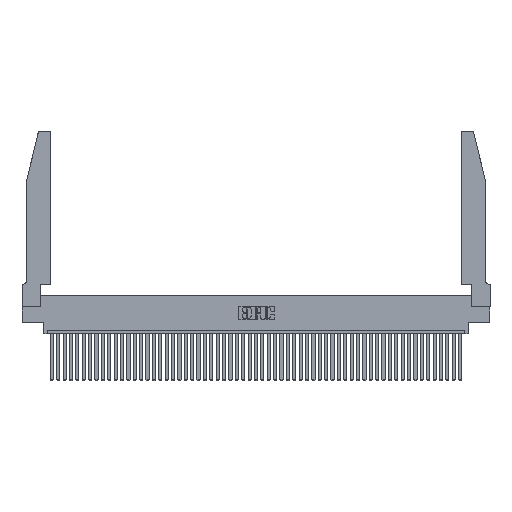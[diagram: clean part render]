
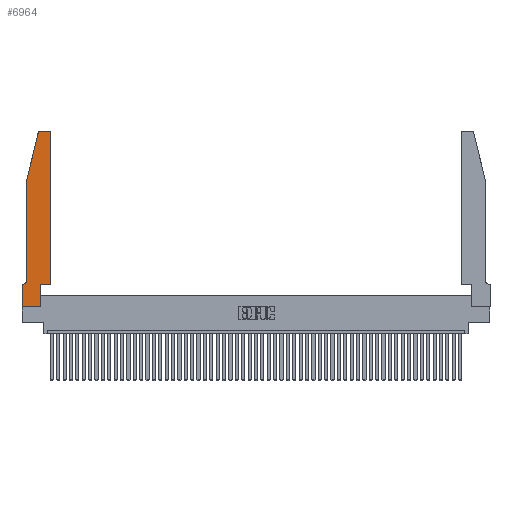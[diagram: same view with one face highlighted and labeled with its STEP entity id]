
A CAD part, top view. The second image highlights one B-rep face of the part: STEP entity #6964.
In plain terms, the highlighted planar face has unit normal (0, 0, 1).
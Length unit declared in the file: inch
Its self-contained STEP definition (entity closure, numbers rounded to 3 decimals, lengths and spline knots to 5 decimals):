
#1527 = DIRECTION ( 'NONE',  ( 0., 1., 0. ) ) ;
#1650 = CARTESIAN_POINT ( 'NONE',  ( 0.2605, 2.75, 0.37 ) ) ;
#1652 = CARTESIAN_POINT ( 'NONE',  ( 0.2865, 0.35, 0.37 ) ) ;
#4080 = VERTEX_POINT ( 'NONE', #32433 ) ;
#4456 = LINE ( 'NONE', #1652, #39812 ) ;
#5148 = CARTESIAN_POINT ( 'NONE',  ( 0., 0., 0.37 ) ) ;
#5754 = EDGE_CURVE ( 'NONE', #23279, #21709, #27894, .T. ) ;
#6207 = CARTESIAN_POINT ( 'NONE',  ( 0.0055, 0.35, 0.37 ) ) ;
#6964 = ADVANCED_FACE ( 'NONE', ( #22169 ), #35498, .T. ) ;
#7252 = VERTEX_POINT ( 'NONE', #6207 ) ;
#7610 = CARTESIAN_POINT ( 'NONE',  ( 0.0755, 2., 0.37 ) ) ;
#8120 = LINE ( 'NONE', #5148, #44692 ) ;
#9779 = VERTEX_POINT ( 'NONE', #18136 ) ;
#9896 = LINE ( 'NONE', #1650, #31781 ) ;
#10762 = VERTEX_POINT ( 'NONE', #33811 ) ;
#10920 = VERTEX_POINT ( 'NONE', #19626 ) ;
#11100 = VERTEX_POINT ( 'NONE', #49220 ) ;
#11203 = DIRECTION ( 'NONE',  ( -0.239, -0.971, 0. ) ) ;
#11654 = VECTOR ( 'NONE', #16954, 39.37008 ) ;
#11927 = CARTESIAN_POINT ( 'NONE',  ( 0.4505, 0.35, 0.37 ) ) ;
#12355 = VECTOR ( 'NONE', #30976, 39.37008 ) ;
#12578 = CARTESIAN_POINT ( 'NONE',  ( 0.0755, 0.35, 0.37 ) ) ;
#13066 = EDGE_CURVE ( 'NONE', #10920, #11100, #47087, .T. ) ;
#13145 = EDGE_CURVE ( 'NONE', #11100, #16964, #33066, .T. ) ;
#13948 = CIRCLE ( 'NONE', #41831, 0.07 ) ;
#14641 = ORIENTED_EDGE ( 'NONE', *, *, #19380, .T. ) ;
#15115 = DIRECTION ( 'NONE',  ( 0., 0., 1. ) ) ;
#15312 = LINE ( 'NONE', #50523, #23232 ) ;
#15313 = EDGE_LOOP ( 'NONE', ( #14641, #48145, #34762, #48092, #24814, #31994, #47638, #49936, #45730, #36715, #20495, #25054 ) ) ;
#15328 = EDGE_CURVE ( 'NONE', #36729, #23279, #18245, .T. ) ;
#15390 = DIRECTION ( 'NONE',  ( 1., 0., 0. ) ) ;
#16580 = VERTEX_POINT ( 'NONE', #29327 ) ;
#16954 = DIRECTION ( 'NONE',  ( -1., 0., 0. ) ) ;
#16964 = VERTEX_POINT ( 'NONE', #40694 ) ;
#16965 = CARTESIAN_POINT ( 'NONE',  ( 0.0755, 2., 0.37 ) ) ;
#17704 = CARTESIAN_POINT ( 'NONE',  ( 0.25487, 2.72718, 0.37 ) ) ;
#18136 = CARTESIAN_POINT ( 'NONE',  ( 0.0755, 0.42, 0.37 ) ) ;
#18245 = CIRCLE ( 'NONE', #34165, 0.03 ) ;
#18463 = DIRECTION ( 'NONE',  ( 0., 0., 1. ) ) ;
#19380 = EDGE_CURVE ( 'NONE', #16964, #36729, #9896, .T. ) ;
#19626 = CARTESIAN_POINT ( 'NONE',  ( 0.4505, 0.35, 0.37 ) ) ;
#20127 = DIRECTION ( 'NONE',  ( 1., 0., 0. ) ) ;
#20192 = CARTESIAN_POINT ( 'NONE',  ( 0., 0., 0.37 ) ) ;
#20495 = ORIENTED_EDGE ( 'NONE', *, *, #13066, .T. ) ;
#20554 = CARTESIAN_POINT ( 'NONE',  ( 0.4505, 0.35, 0.37 ) ) ;
#21009 = DIRECTION ( 'NONE',  ( 0., -1., 0. ) ) ;
#21709 = VERTEX_POINT ( 'NONE', #16965 ) ;
#21934 = VERTEX_POINT ( 'NONE', #20192 ) ;
#22025 = LINE ( 'NONE', #12578, #11654 ) ;
#22169 = FACE_OUTER_BOUND ( 'NONE', #15313, .T. ) ;
#23232 = VECTOR ( 'NONE', #15390, 39.37008 ) ;
#23279 = VERTEX_POINT ( 'NONE', #17704 ) ;
#23739 = CARTESIAN_POINT ( 'NONE',  ( 0.0755, 2., 0.37 ) ) ;
#24238 = DIRECTION ( 'NONE',  ( 0., 0., 1. ) ) ;
#24558 = EDGE_CURVE ( 'NONE', #21709, #9779, #44012, .T. ) ;
#24789 = DIRECTION ( 'NONE',  ( 0., 1., 0. ) ) ;
#24814 = ORIENTED_EDGE ( 'NONE', *, *, #33190, .T. ) ;
#25054 = ORIENTED_EDGE ( 'NONE', *, *, #13145, .T. ) ;
#25460 = VECTOR ( 'NONE', #11203, 39.37008 ) ;
#26662 = DIRECTION ( 'NONE',  ( 1., 0., 0. ) ) ;
#27894 = LINE ( 'NONE', #7610, #25460 ) ;
#27933 = EDGE_CURVE ( 'NONE', #16580, #21934, #8120, .T. ) ;
#28600 = CARTESIAN_POINT ( 'NONE',  ( 0.284, 2.75, 0.37 ) ) ;
#29327 = CARTESIAN_POINT ( 'NONE',  ( 0., 0.35, 0.37 ) ) ;
#30168 = EDGE_CURVE ( 'NONE', #7252, #16580, #22025, .T. ) ;
#30976 = DIRECTION ( 'NONE',  ( 0., -1., 0. ) ) ;
#31781 = VECTOR ( 'NONE', #33511, 39.37008 ) ;
#31969 = EDGE_CURVE ( 'NONE', #21934, #4080, #15312, .T. ) ;
#31994 = ORIENTED_EDGE ( 'NONE', *, *, #30168, .T. ) ;
#32019 = DIRECTION ( 'NONE',  ( 1., 0., 0. ) ) ;
#32433 = CARTESIAN_POINT ( 'NONE',  ( 0.2865, 0., 0.37 ) ) ;
#33066 = CIRCLE ( 'NONE', #35209, 0.03 ) ;
#33190 = EDGE_CURVE ( 'NONE', #9779, #7252, #13948, .T. ) ;
#33511 = DIRECTION ( 'NONE',  ( -1., 0., 0. ) ) ;
#33811 = CARTESIAN_POINT ( 'NONE',  ( 0.2865, 0.35, 0.37 ) ) ;
#34165 = AXIS2_PLACEMENT_3D ( 'NONE', #38631, #15115, #41172 ) ;
#34414 = AXIS2_PLACEMENT_3D ( 'NONE', #44010, #24238, #20127 ) ;
#34762 = ORIENTED_EDGE ( 'NONE', *, *, #5754, .T. ) ;
#35209 = AXIS2_PLACEMENT_3D ( 'NONE', #38238, #18463, #26662 ) ;
#35256 = DIRECTION ( 'NONE',  ( 0., 0., -1. ) ) ;
#35498 = PLANE ( 'NONE',  #34414 ) ;
#36715 = ORIENTED_EDGE ( 'NONE', *, *, #47033, .T. ) ;
#36729 = VERTEX_POINT ( 'NONE', #28600 ) ;
#38238 = CARTESIAN_POINT ( 'NONE',  ( 0.4205, 2.72, 0.37 ) ) ;
#38531 = VECTOR ( 'NONE', #32019, 39.37008 ) ;
#38631 = CARTESIAN_POINT ( 'NONE',  ( 0.284, 2.72, 0.37 ) ) ;
#39679 = CARTESIAN_POINT ( 'NONE',  ( 0.0055, 0.42, 0.37 ) ) ;
#39812 = VECTOR ( 'NONE', #24789, 39.37008 ) ;
#40452 = EDGE_CURVE ( 'NONE', #4080, #10762, #4456, .T. ) ;
#40694 = CARTESIAN_POINT ( 'NONE',  ( 0.4205, 2.75, 0.37 ) ) ;
#41172 = DIRECTION ( 'NONE',  ( 1., 0., 0. ) ) ;
#41831 = AXIS2_PLACEMENT_3D ( 'NONE', #39679, #35256, #43599 ) ;
#43599 = DIRECTION ( 'NONE',  ( -1., 0., 0. ) ) ;
#44010 = CARTESIAN_POINT ( 'NONE',  ( 0., 0.35, 0.37 ) ) ;
#44012 = LINE ( 'NONE', #23739, #12355 ) ;
#44692 = VECTOR ( 'NONE', #21009, 39.37008 ) ;
#45730 = ORIENTED_EDGE ( 'NONE', *, *, #40452, .T. ) ;
#45886 = VECTOR ( 'NONE', #1527, 39.37008 ) ;
#46453 = LINE ( 'NONE', #20554, #38531 ) ;
#47033 = EDGE_CURVE ( 'NONE', #10762, #10920, #46453, .T. ) ;
#47087 = LINE ( 'NONE', #11927, #45886 ) ;
#47638 = ORIENTED_EDGE ( 'NONE', *, *, #27933, .T. ) ;
#48092 = ORIENTED_EDGE ( 'NONE', *, *, #24558, .T. ) ;
#48145 = ORIENTED_EDGE ( 'NONE', *, *, #15328, .T. ) ;
#49220 = CARTESIAN_POINT ( 'NONE',  ( 0.4505, 2.72, 0.37 ) ) ;
#49936 = ORIENTED_EDGE ( 'NONE', *, *, #31969, .T. ) ;
#50523 = CARTESIAN_POINT ( 'NONE',  ( 0., 0., 0.37 ) ) ;
